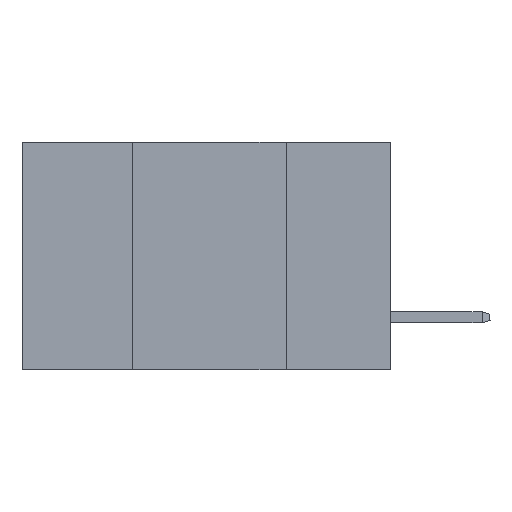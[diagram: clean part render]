
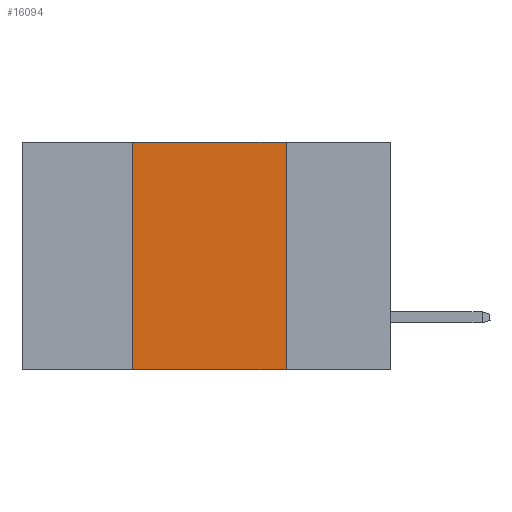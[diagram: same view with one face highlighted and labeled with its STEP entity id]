
A CAD part, left-side view. The second image highlights one B-rep face of the part: STEP entity #16094.
In plain terms, the highlighted planar face has unit normal (-1, 0, 0).
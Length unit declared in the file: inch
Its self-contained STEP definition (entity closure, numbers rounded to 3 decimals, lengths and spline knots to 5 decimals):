
#997 = VERTEX_POINT ( 'NONE', #5345 ) ;
#1159 = DIRECTION ( 'NONE',  ( 0., -1., 0. ) ) ;
#1942 = EDGE_LOOP ( 'NONE', ( #12027, #5587, #9474, #16342 ) ) ;
#2193 = VECTOR ( 'NONE', #10234, 39.37008 ) ;
#2384 = CARTESIAN_POINT ( 'NONE',  ( 0., 0.17, 0. ) ) ;
#2750 = VERTEX_POINT ( 'NONE', #5972 ) ;
#2969 = LINE ( 'NONE', #13651, #14826 ) ;
#3791 = PLANE ( 'NONE',  #9488 ) ;
#4125 = CARTESIAN_POINT ( 'NONE',  ( 0., 0.6, 0. ) ) ;
#4305 = FACE_OUTER_BOUND ( 'NONE', #1942, .T. ) ;
#4621 = VERTEX_POINT ( 'NONE', #7872 ) ;
#4678 = CARTESIAN_POINT ( 'NONE',  ( 0., 0.42, 0. ) ) ;
#5035 = LINE ( 'NONE', #17448, #18019 ) ;
#5345 = CARTESIAN_POINT ( 'NONE',  ( 0., 0.17, 0. ) ) ;
#5587 = ORIENTED_EDGE ( 'NONE', *, *, #11997, .F. ) ;
#5972 = CARTESIAN_POINT ( 'NONE',  ( 0., 0.42, 0. ) ) ;
#6409 = EDGE_CURVE ( 'NONE', #997, #13757, #8873, .T. ) ;
#7063 = CARTESIAN_POINT ( 'NONE',  ( 0., 0.17, -0.37 ) ) ;
#7872 = CARTESIAN_POINT ( 'NONE',  ( 0., 0.42, -0.37 ) ) ;
#8873 = LINE ( 'NONE', #2384, #10198 ) ;
#9474 = ORIENTED_EDGE ( 'NONE', *, *, #10774, .F. ) ;
#9488 = AXIS2_PLACEMENT_3D ( 'NONE', #4125, #16897, #12512 ) ;
#10198 = VECTOR ( 'NONE', #16240, 39.37008 ) ;
#10234 = DIRECTION ( 'NONE',  ( 0., 0., 1. ) ) ;
#10774 = EDGE_CURVE ( 'NONE', #4621, #2750, #14524, .T. ) ;
#11997 = EDGE_CURVE ( 'NONE', #2750, #997, #2969, .T. ) ;
#12027 = ORIENTED_EDGE ( 'NONE', *, *, #6409, .F. ) ;
#12512 = DIRECTION ( 'NONE',  ( 0., 0., -1. ) ) ;
#13651 = CARTESIAN_POINT ( 'NONE',  ( 0., 0.6, 0. ) ) ;
#13757 = VERTEX_POINT ( 'NONE', #7063 ) ;
#13987 = EDGE_CURVE ( 'NONE', #4621, #13757, #5035, .T. ) ;
#14524 = LINE ( 'NONE', #4678, #2193 ) ;
#14826 = VECTOR ( 'NONE', #1159, 39.37008 ) ;
#15982 = DIRECTION ( 'NONE',  ( 0., -1., 0. ) ) ;
#16094 = ADVANCED_FACE ( 'NONE', ( #4305 ), #3791, .F. ) ;
#16240 = DIRECTION ( 'NONE',  ( 0., 0., -1. ) ) ;
#16342 = ORIENTED_EDGE ( 'NONE', *, *, #13987, .T. ) ;
#16897 = DIRECTION ( 'NONE',  ( 1., 0., 0. ) ) ;
#17448 = CARTESIAN_POINT ( 'NONE',  ( 0., 0.6, -0.37 ) ) ;
#18019 = VECTOR ( 'NONE', #15982, 39.37008 ) ;
